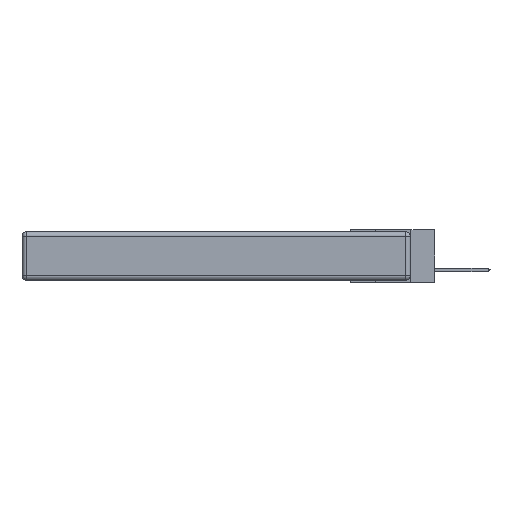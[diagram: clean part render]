
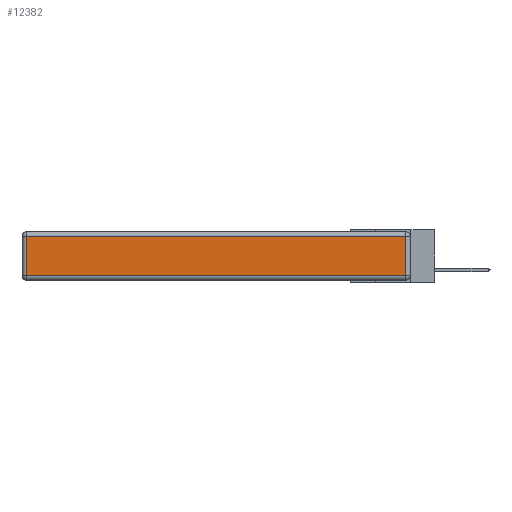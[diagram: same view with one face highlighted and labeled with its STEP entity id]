
A CAD part, left-side view. The second image highlights one B-rep face of the part: STEP entity #12382.
In plain terms, the highlighted planar face has unit normal (-1, 0, 0).
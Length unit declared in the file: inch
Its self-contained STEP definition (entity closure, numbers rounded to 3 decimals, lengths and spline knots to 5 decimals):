
#54 = DIRECTION ( 'NONE',  ( 0., 1., 0. ) ) ;
#345 = LINE ( 'NONE', #13888, #6620 ) ;
#1488 = ORIENTED_EDGE ( 'NONE', *, *, #10981, .T. ) ;
#1686 = VECTOR ( 'NONE', #13647, 39.37008 ) ;
#2172 = LINE ( 'NONE', #11811, #6481 ) ;
#2206 = CARTESIAN_POINT ( 'NONE',  ( 0., 0., -0.343 ) ) ;
#2396 = CARTESIAN_POINT ( 'NONE',  ( 0., 2.72, -0.313 ) ) ;
#2758 = CARTESIAN_POINT ( 'NONE',  ( 0., 2.72, -0.343 ) ) ;
#3202 = ORIENTED_EDGE ( 'NONE', *, *, #6361, .T. ) ;
#3548 = DIRECTION ( 'NONE',  ( 0., 0., 1. ) ) ;
#3811 = EDGE_CURVE ( 'NONE', #16164, #11160, #8376, .T. ) ;
#3909 = CARTESIAN_POINT ( 'NONE',  ( 0., 0.03, -0.03 ) ) ;
#4296 = DIRECTION ( 'NONE',  ( 0., 0., 1. ) ) ;
#4499 = ORIENTED_EDGE ( 'NONE', *, *, #3811, .T. ) ;
#4816 = CARTESIAN_POINT ( 'NONE',  ( 0., 0., -0.313 ) ) ;
#5522 = VERTEX_POINT ( 'NONE', #3909 ) ;
#6361 = EDGE_CURVE ( 'NONE', #11888, #16164, #8319, .T. ) ;
#6481 = VECTOR ( 'NONE', #4296, 39.37008 ) ;
#6620 = VECTOR ( 'NONE', #54, 39.37008 ) ;
#7339 = CARTESIAN_POINT ( 'NONE',  ( 0., 0.03, -0.313 ) ) ;
#8319 = LINE ( 'NONE', #2758, #15445 ) ;
#8376 = LINE ( 'NONE', #4816, #1686 ) ;
#8612 = EDGE_LOOP ( 'NONE', ( #4499, #1488, #13196, #3202 ) ) ;
#9123 = EDGE_CURVE ( 'NONE', #5522, #11888, #345, .T. ) ;
#10981 = EDGE_CURVE ( 'NONE', #11160, #5522, #2172, .T. ) ;
#10987 = DIRECTION ( 'NONE',  ( -1., 0., 0. ) ) ;
#11160 = VERTEX_POINT ( 'NONE', #7339 ) ;
#11214 = PLANE ( 'NONE',  #13766 ) ;
#11811 = CARTESIAN_POINT ( 'NONE',  ( 0., 0.03, -0.343 ) ) ;
#11888 = VERTEX_POINT ( 'NONE', #12398 ) ;
#12382 = ADVANCED_FACE ( 'NONE', ( #14367 ), #11214, .T. ) ;
#12398 = CARTESIAN_POINT ( 'NONE',  ( 0., 2.72, -0.03 ) ) ;
#13196 = ORIENTED_EDGE ( 'NONE', *, *, #9123, .T. ) ;
#13647 = DIRECTION ( 'NONE',  ( 0., -1., 0. ) ) ;
#13766 = AXIS2_PLACEMENT_3D ( 'NONE', #2206, #10987, #3548 ) ;
#13888 = CARTESIAN_POINT ( 'NONE',  ( 0., 2.75, -0.03 ) ) ;
#13945 = DIRECTION ( 'NONE',  ( 0., 0., -1. ) ) ;
#14367 = FACE_OUTER_BOUND ( 'NONE', #8612, .T. ) ;
#15445 = VECTOR ( 'NONE', #13945, 39.37008 ) ;
#16164 = VERTEX_POINT ( 'NONE', #2396 ) ;
